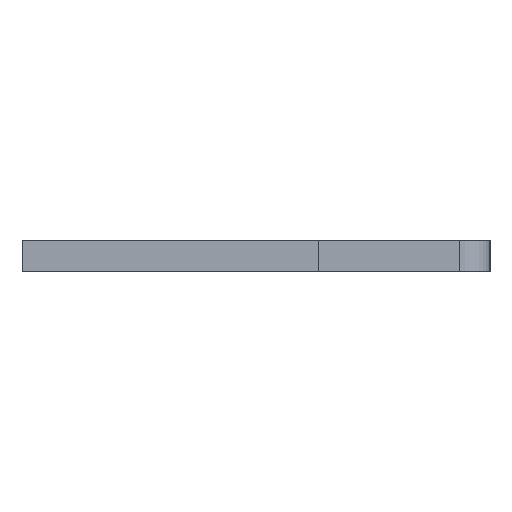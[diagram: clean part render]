
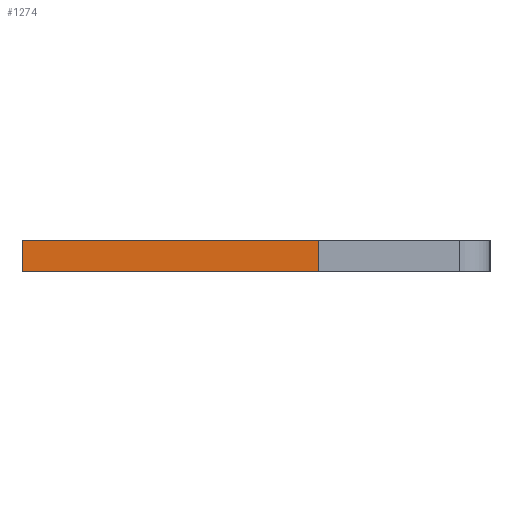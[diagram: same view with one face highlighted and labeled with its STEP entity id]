
A CAD part, left-side view. The second image highlights one B-rep face of the part: STEP entity #1274.
In plain terms, the highlighted face is planar.
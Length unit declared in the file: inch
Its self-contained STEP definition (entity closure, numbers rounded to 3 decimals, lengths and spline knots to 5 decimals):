
#14 = LINE ( 'NONE', #890, #2219 ) ;
#60 = DIRECTION ( 'NONE',  ( 0., 1., 0. ) ) ;
#157 = CARTESIAN_POINT ( 'NONE',  ( 0.01, 0.15, -0.04 ) ) ;
#176 = DIRECTION ( 'NONE',  ( 0., 0., 1. ) ) ;
#211 = CARTESIAN_POINT ( 'NONE',  ( 0.01, -0.04, -0.04 ) ) ;
#267 = CARTESIAN_POINT ( 'NONE',  ( 0.01, -0.04, -0.04 ) ) ;
#286 = CARTESIAN_POINT ( 'NONE',  ( -0.01, 0.15, -0.04 ) ) ;
#360 = DIRECTION ( 'NONE',  ( 0., 1., 0. ) ) ;
#422 = VECTOR ( 'NONE', #979, 39.37008 ) ;
#507 = LINE ( 'NONE', #267, #422 ) ;
#533 = VECTOR ( 'NONE', #60, 39.37008 ) ;
#735 = FACE_OUTER_BOUND ( 'NONE', #2003, .T. ) ;
#767 = VERTEX_POINT ( 'NONE', #1095 ) ;
#834 = ORIENTED_EDGE ( 'NONE', *, *, #1081, .F. ) ;
#890 = CARTESIAN_POINT ( 'NONE',  ( 0.01, 0.15, -0.04 ) ) ;
#906 = VERTEX_POINT ( 'NONE', #286 ) ;
#910 = CARTESIAN_POINT ( 'NONE',  ( 0.01, 0.15, -0.04 ) ) ;
#979 = DIRECTION ( 'NONE',  ( -1., 0., 0. ) ) ;
#1012 = VERTEX_POINT ( 'NONE', #157 ) ;
#1039 = EDGE_CURVE ( 'NONE', #1107, #767, #507, .T. ) ;
#1081 = EDGE_CURVE ( 'NONE', #1107, #1012, #14, .T. ) ;
#1095 = CARTESIAN_POINT ( 'NONE',  ( -0.01, -0.04, -0.04 ) ) ;
#1107 = VERTEX_POINT ( 'NONE', #211 ) ;
#1135 = ORIENTED_EDGE ( 'NONE', *, *, #1039, .T. ) ;
#1274 = ADVANCED_FACE ( 'NONE', ( #735 ), #1608, .F. ) ;
#1454 = DIRECTION ( 'NONE',  ( 1., 0., 0. ) ) ;
#1608 = PLANE ( 'NONE',  #1854 ) ;
#1628 = ORIENTED_EDGE ( 'NONE', *, *, #1832, .F. ) ;
#1664 = DIRECTION ( 'NONE',  ( -1., 0., 0. ) ) ;
#1832 = EDGE_CURVE ( 'NONE', #1012, #906, #2126, .T. ) ;
#1854 = AXIS2_PLACEMENT_3D ( 'NONE', #910, #176, #1454 ) ;
#1876 = CARTESIAN_POINT ( 'NONE',  ( 0.01, 0.15, -0.04 ) ) ;
#1923 = ORIENTED_EDGE ( 'NONE', *, *, #2227, .T. ) ;
#2003 = EDGE_LOOP ( 'NONE', ( #1923, #1628, #834, #1135 ) ) ;
#2075 = VECTOR ( 'NONE', #1664, 39.37008 ) ;
#2126 = LINE ( 'NONE', #1876, #2075 ) ;
#2219 = VECTOR ( 'NONE', #360, 39.37008 ) ;
#2227 = EDGE_CURVE ( 'NONE', #767, #906, #2247, .T. ) ;
#2247 = LINE ( 'NONE', #2255, #533 ) ;
#2255 = CARTESIAN_POINT ( 'NONE',  ( -0.01, 0.15, -0.04 ) ) ;
